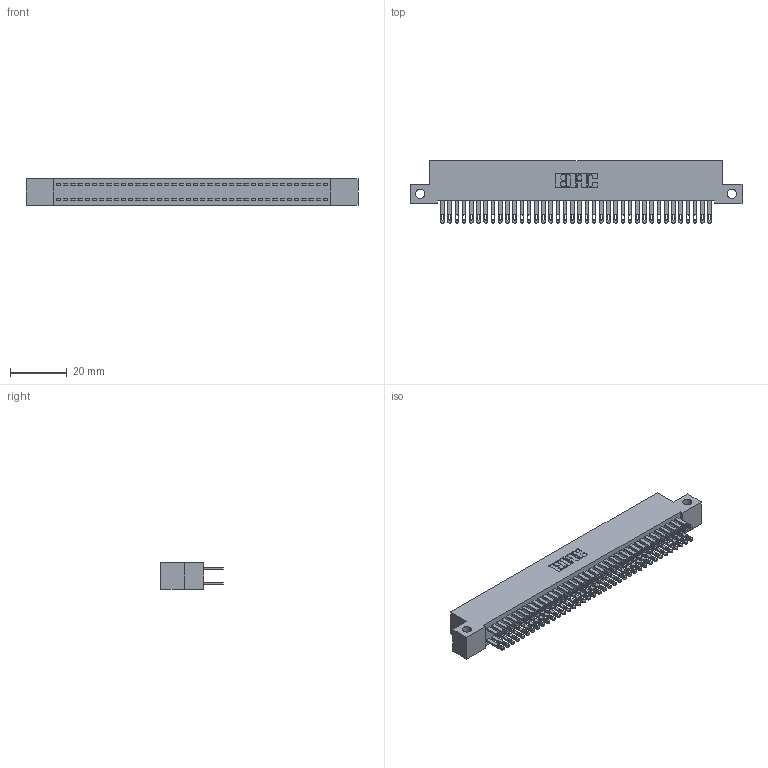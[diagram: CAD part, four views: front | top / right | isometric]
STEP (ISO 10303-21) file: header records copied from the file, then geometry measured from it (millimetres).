
FILE_DESCRIPTION (( 'STEP AP203' ), '1' );
FILE_NAME ('892-076-500-212.STEP', '2020-09-21T20:02:02', ( '' ), ( '' ), 'SwSTEP 2.0', 'SolidWorks 2020', '' );
FILE_SCHEMA (( 'CONFIG_CONTROL_DESIGN' ));
Length unit declared in the file: inch
Products named in the file (3): 842 Part_Side Mount; 345-292-001_345-293-100; 892-076-500-212
Assembly tree (77 placements, depth 2):
  892-076-500-212
    842 Part_Side Mount
    345-292-001_345-293-100  x76
Bounding box: 116.84 x 21.85 x 9.4 mm (x, y, z)
Volume: 10637.4 mm3; surface area: 17784.4 mm2
Topology: 77 solids, 77 shells, 3758 faces, 11471 edges, 7646 vertices
Faces by surface type: plane 2346, cylinder 1412
Entity records: 24765 total; most frequent: CARTESIAN_POINT 4106, ORIENTED_EDGE 4042, DIRECTION 3517, EDGE_CURVE 2021, VECTOR 1889, LINE 1889, VERTEX_POINT 1346, AXIS2_PLACEMENT_3D 814
